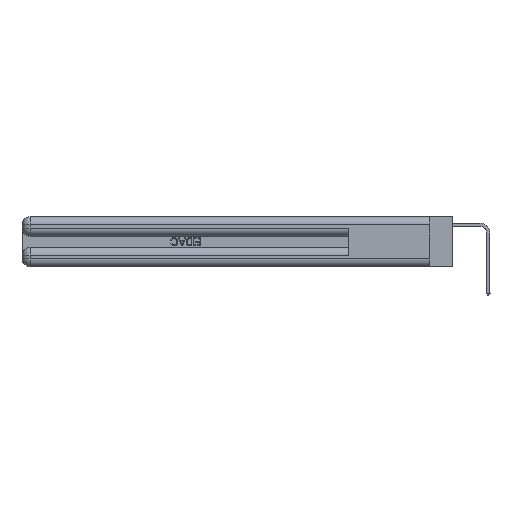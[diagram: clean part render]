
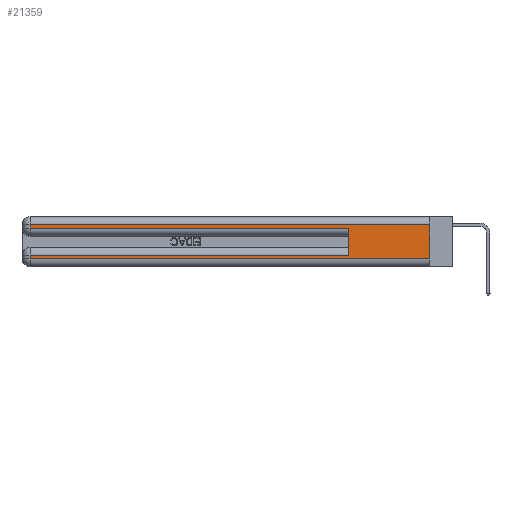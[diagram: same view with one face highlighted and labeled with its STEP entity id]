
A CAD part, left-side view. The second image highlights one B-rep face of the part: STEP entity #21359.
In plain terms, the highlighted planar face has unit normal (-1, 0, 0).
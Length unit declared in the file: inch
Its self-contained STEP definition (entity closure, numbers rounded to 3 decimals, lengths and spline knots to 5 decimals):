
#176 = CARTESIAN_POINT ( 'NONE',  ( 0., 0., 0.37 ) ) ;
#1065 = CARTESIAN_POINT ( 'NONE',  ( 0., 2.94, 0.06 ) ) ;
#1513 = DIRECTION ( 'NONE',  ( 0., -1., 0. ) ) ;
#2610 = DIRECTION ( 'NONE',  ( 0., 0., -1. ) ) ;
#2978 = DIRECTION ( 'NONE',  ( 0., 0., 1. ) ) ;
#4451 = FACE_OUTER_BOUND ( 'NONE', #20474, .T. ) ;
#4799 = VERTEX_POINT ( 'NONE', #1065 ) ;
#4812 = LINE ( 'NONE', #7702, #13621 ) ;
#4832 = CARTESIAN_POINT ( 'NONE',  ( 0., 2.94, 0.37 ) ) ;
#5621 = VERTEX_POINT ( 'NONE', #22336 ) ;
#6117 = CARTESIAN_POINT ( 'NONE',  ( 0., 0., 0.37 ) ) ;
#7190 = VECTOR ( 'NONE', #17966, 39.37008 ) ;
#7270 = LINE ( 'NONE', #4832, #27495 ) ;
#7564 = VERTEX_POINT ( 'NONE', #12595 ) ;
#7661 = VERTEX_POINT ( 'NONE', #22957 ) ;
#7702 = CARTESIAN_POINT ( 'NONE',  ( 0., 0.6, 0.145 ) ) ;
#8355 = LINE ( 'NONE', #22254, #16348 ) ;
#8766 = LINE ( 'NONE', #26773, #7190 ) ;
#9287 = CARTESIAN_POINT ( 'NONE',  ( 0., 0.6, 0.085 ) ) ;
#9415 = VERTEX_POINT ( 'NONE', #25096 ) ;
#9494 = EDGE_CURVE ( 'NONE', #9751, #14570, #4812, .T. ) ;
#9751 = VERTEX_POINT ( 'NONE', #9287 ) ;
#9790 = DIRECTION ( 'NONE',  ( 0., -1., 0. ) ) ;
#11582 = CARTESIAN_POINT ( 'NONE',  ( 0., 2.94, 0.285 ) ) ;
#11758 = LINE ( 'NONE', #27644, #27099 ) ;
#11857 = LINE ( 'NONE', #176, #15019 ) ;
#12012 = ORIENTED_EDGE ( 'NONE', *, *, #15795, .T. ) ;
#12391 = VERTEX_POINT ( 'NONE', #11582 ) ;
#12595 = CARTESIAN_POINT ( 'NONE',  ( 0., 0., 0.31 ) ) ;
#12704 = LINE ( 'NONE', #12842, #18990 ) ;
#12842 = CARTESIAN_POINT ( 'NONE',  ( 0., 0., 0.085 ) ) ;
#12903 = EDGE_CURVE ( 'NONE', #7661, #4799, #7270, .T. ) ;
#13621 = VECTOR ( 'NONE', #2978, 39.37008 ) ;
#13692 = PLANE ( 'NONE',  #21348 ) ;
#14271 = DIRECTION ( 'NONE',  ( 0., 0., -1. ) ) ;
#14570 = VERTEX_POINT ( 'NONE', #27250 ) ;
#14654 = DIRECTION ( 'NONE',  ( 0., 0., -1. ) ) ;
#14972 = ORIENTED_EDGE ( 'NONE', *, *, #12903, .T. ) ;
#15019 = VECTOR ( 'NONE', #14271, 39.37008 ) ;
#15795 = EDGE_CURVE ( 'NONE', #5621, #12391, #8766, .T. ) ;
#16348 = VECTOR ( 'NONE', #1513, 39.37008 ) ;
#17153 = EDGE_CURVE ( 'NONE', #4799, #9415, #8355, .T. ) ;
#17268 = CARTESIAN_POINT ( 'NONE',  ( 0., 0., 0.31 ) ) ;
#17966 = DIRECTION ( 'NONE',  ( 0., 0., -1. ) ) ;
#18354 = EDGE_CURVE ( 'NONE', #7564, #5621, #26529, .T. ) ;
#18423 = ORIENTED_EDGE ( 'NONE', *, *, #20377, .F. ) ;
#18990 = VECTOR ( 'NONE', #19618, 39.37008 ) ;
#19528 = ORIENTED_EDGE ( 'NONE', *, *, #18354, .T. ) ;
#19618 = DIRECTION ( 'NONE',  ( 0., 1., 0. ) ) ;
#19981 = EDGE_CURVE ( 'NONE', #12391, #14570, #11758, .T. ) ;
#20377 = EDGE_CURVE ( 'NONE', #7564, #9415, #11857, .T. ) ;
#20474 = EDGE_LOOP ( 'NONE', ( #18423, #19528, #12012, #25035, #25742, #29063, #14972, #27417 ) ) ;
#20725 = VECTOR ( 'NONE', #26674, 39.37008 ) ;
#21348 = AXIS2_PLACEMENT_3D ( 'NONE', #6117, #23361, #2610 ) ;
#21359 = ADVANCED_FACE ( 'NONE', ( #4451 ), #13692, .F. ) ;
#22254 = CARTESIAN_POINT ( 'NONE',  ( 0., 0., 0.06 ) ) ;
#22336 = CARTESIAN_POINT ( 'NONE',  ( 0., 2.94, 0.31 ) ) ;
#22957 = CARTESIAN_POINT ( 'NONE',  ( 0., 2.94, 0.085 ) ) ;
#23361 = DIRECTION ( 'NONE',  ( 1., 0., 0. ) ) ;
#24283 = EDGE_CURVE ( 'NONE', #9751, #7661, #12704, .T. ) ;
#25035 = ORIENTED_EDGE ( 'NONE', *, *, #19981, .T. ) ;
#25096 = CARTESIAN_POINT ( 'NONE',  ( 0., 0., 0.06 ) ) ;
#25742 = ORIENTED_EDGE ( 'NONE', *, *, #9494, .F. ) ;
#26529 = LINE ( 'NONE', #17268, #20725 ) ;
#26674 = DIRECTION ( 'NONE',  ( 0., 1., 0. ) ) ;
#26773 = CARTESIAN_POINT ( 'NONE',  ( 0., 2.94, 0.37 ) ) ;
#27099 = VECTOR ( 'NONE', #9790, 39.37008 ) ;
#27250 = CARTESIAN_POINT ( 'NONE',  ( 0., 0.6, 0.285 ) ) ;
#27417 = ORIENTED_EDGE ( 'NONE', *, *, #17153, .T. ) ;
#27495 = VECTOR ( 'NONE', #14654, 39.37008 ) ;
#27644 = CARTESIAN_POINT ( 'NONE',  ( 0., 0., 0.285 ) ) ;
#29063 = ORIENTED_EDGE ( 'NONE', *, *, #24283, .T. ) ;
